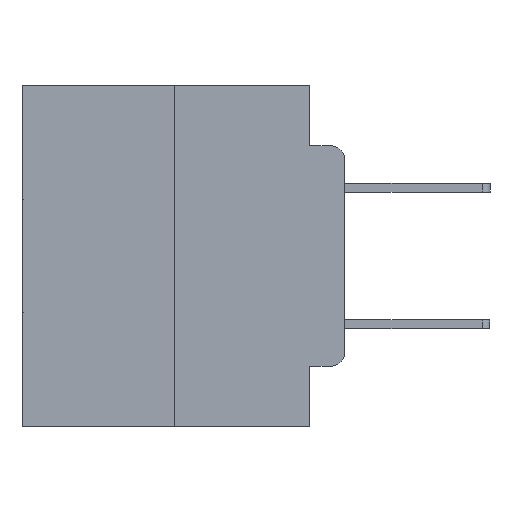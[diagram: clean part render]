
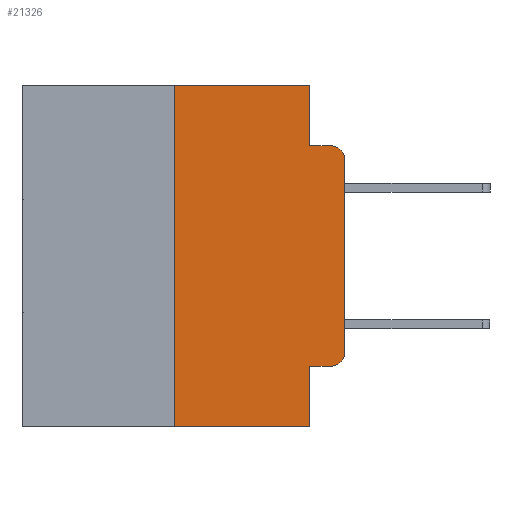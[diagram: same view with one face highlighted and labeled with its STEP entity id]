
A CAD part, left-side view. The second image highlights one B-rep face of the part: STEP entity #21326.
In plain terms, the highlighted planar face has unit normal (-1, 0, 0).
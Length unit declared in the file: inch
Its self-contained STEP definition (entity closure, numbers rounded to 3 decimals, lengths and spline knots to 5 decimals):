
#65 = VECTOR ( 'NONE', #10682, 39.37008 ) ;
#581 = AXIS2_PLACEMENT_3D ( 'NONE', #2863, #18150, #5089 ) ;
#808 = CARTESIAN_POINT ( 'NONE',  ( 0., 0.02, -0.0885 ) ) ;
#842 = CARTESIAN_POINT ( 'NONE',  ( 0., 0.473, 0. ) ) ;
#845 = CARTESIAN_POINT ( 'NONE',  ( 0., 0.051, -0.0885 ) ) ;
#1761 = LINE ( 'NONE', #6382, #12004 ) ;
#1938 = ORIENTED_EDGE ( 'NONE', *, *, #10150, .F. ) ;
#2787 = DIRECTION ( 'NONE',  ( 0., -1., 0. ) ) ;
#2863 = CARTESIAN_POINT ( 'NONE',  ( 0., 0.02, -0.1085 ) ) ;
#3636 = VECTOR ( 'NONE', #24795, 39.37008 ) ;
#4449 = AXIS2_PLACEMENT_3D ( 'NONE', #5507, #20698, #7735 ) ;
#4589 = CARTESIAN_POINT ( 'NONE',  ( 0., 0., -0.3915 ) ) ;
#4652 = VECTOR ( 'NONE', #23548, 39.37008 ) ;
#4990 = EDGE_LOOP ( 'NONE', ( #17980, #5384, #1938, #7462, #9642, #26324, #7247, #12458, #26507, #12456 ) ) ;
#5089 = DIRECTION ( 'NONE',  ( 0., 0., -1. ) ) ;
#5300 = DIRECTION ( 'NONE',  ( 1., 0., 0. ) ) ;
#5384 = ORIENTED_EDGE ( 'NONE', *, *, #11597, .T. ) ;
#5507 = CARTESIAN_POINT ( 'NONE',  ( 0., 0.02, -0.3915 ) ) ;
#5779 = EDGE_CURVE ( 'NONE', #7397, #6292, #14840, .T. ) ;
#6292 = VERTEX_POINT ( 'NONE', #16564 ) ;
#6382 = CARTESIAN_POINT ( 'NONE',  ( 0., 0.473, -0.5 ) ) ;
#6900 = FACE_OUTER_BOUND ( 'NONE', #4990, .T. ) ;
#7247 = ORIENTED_EDGE ( 'NONE', *, *, #27016, .T. ) ;
#7397 = VERTEX_POINT ( 'NONE', #4589 ) ;
#7462 = ORIENTED_EDGE ( 'NONE', *, *, #11059, .F. ) ;
#7468 = DIRECTION ( 'NONE',  ( 0., 0., -1. ) ) ;
#7735 = DIRECTION ( 'NONE',  ( 0., 0., -1. ) ) ;
#8162 = VERTEX_POINT ( 'NONE', #11387 ) ;
#8421 = CARTESIAN_POINT ( 'NONE',  ( 0., 0., 0. ) ) ;
#9582 = PLANE ( 'NONE',  #23136 ) ;
#9642 = ORIENTED_EDGE ( 'NONE', *, *, #26038, .F. ) ;
#9978 = VECTOR ( 'NONE', #7468, 39.37008 ) ;
#10150 = EDGE_CURVE ( 'NONE', #20978, #27968, #14664, .T. ) ;
#10536 = CIRCLE ( 'NONE', #4449, 0.02 ) ;
#10682 = DIRECTION ( 'NONE',  ( 0., -1., 0. ) ) ;
#10781 = VERTEX_POINT ( 'NONE', #15310 ) ;
#11052 = LINE ( 'NONE', #25806, #65 ) ;
#11059 = EDGE_CURVE ( 'NONE', #8162, #20978, #19722, .T. ) ;
#11387 = CARTESIAN_POINT ( 'NONE',  ( 0., 0.051, 0. ) ) ;
#11597 = EDGE_CURVE ( 'NONE', #6292, #27968, #12543, .T. ) ;
#11828 = CARTESIAN_POINT ( 'NONE',  ( 0., 0.25, 0. ) ) ;
#12004 = VECTOR ( 'NONE', #25868, 39.37008 ) ;
#12456 = ORIENTED_EDGE ( 'NONE', *, *, #22674, .T. ) ;
#12458 = ORIENTED_EDGE ( 'NONE', *, *, #19800, .F. ) ;
#12543 = CIRCLE ( 'NONE', #581, 0.02 ) ;
#13041 = EDGE_CURVE ( 'NONE', #10781, #26845, #20321, .T. ) ;
#13046 = DIRECTION ( 'NONE',  ( 0., -1., 0. ) ) ;
#13272 = VERTEX_POINT ( 'NONE', #19242 ) ;
#14606 = VECTOR ( 'NONE', #26967, 39.37008 ) ;
#14664 = LINE ( 'NONE', #15153, #25472 ) ;
#14840 = LINE ( 'NONE', #8421, #4652 ) ;
#15153 = CARTESIAN_POINT ( 'NONE',  ( 0., 0.051, -0.0885 ) ) ;
#15310 = CARTESIAN_POINT ( 'NONE',  ( 0., 0.25, -0.5 ) ) ;
#15766 = LINE ( 'NONE', #20454, #9978 ) ;
#16564 = CARTESIAN_POINT ( 'NONE',  ( 0., 0., -0.1085 ) ) ;
#17858 = CARTESIAN_POINT ( 'NONE',  ( 0., 0.051, -0.4115 ) ) ;
#17980 = ORIENTED_EDGE ( 'NONE', *, *, #5779, .T. ) ;
#18150 = DIRECTION ( 'NONE',  ( -1., 0., 0. ) ) ;
#19242 = CARTESIAN_POINT ( 'NONE',  ( 0., 0.02, -0.4115 ) ) ;
#19722 = LINE ( 'NONE', #24822, #14606 ) ;
#19795 = VECTOR ( 'NONE', #2787, 39.37008 ) ;
#19800 = EDGE_CURVE ( 'NONE', #27847, #20444, #15766, .T. ) ;
#20118 = CARTESIAN_POINT ( 'NONE',  ( 0., 0.051, -0.4115 ) ) ;
#20321 = LINE ( 'NONE', #11828, #3636 ) ;
#20444 = VERTEX_POINT ( 'NONE', #22871 ) ;
#20454 = CARTESIAN_POINT ( 'NONE',  ( 0., 0.051, 0. ) ) ;
#20491 = DIRECTION ( 'NONE',  ( 0., 0., -1. ) ) ;
#20698 = DIRECTION ( 'NONE',  ( -1., 0., 0. ) ) ;
#20978 = VERTEX_POINT ( 'NONE', #845 ) ;
#21247 = EDGE_CURVE ( 'NONE', #27847, #13272, #25498, .T. ) ;
#21326 = ADVANCED_FACE ( 'NONE', ( #6900 ), #9582, .F. ) ;
#22472 = CARTESIAN_POINT ( 'NONE',  ( 0., 0.25, 0. ) ) ;
#22674 = EDGE_CURVE ( 'NONE', #13272, #7397, #10536, .T. ) ;
#22871 = CARTESIAN_POINT ( 'NONE',  ( 0., 0.051, -0.5 ) ) ;
#23136 = AXIS2_PLACEMENT_3D ( 'NONE', #842, #5300, #20491 ) ;
#23548 = DIRECTION ( 'NONE',  ( 0., 0., 1. ) ) ;
#24795 = DIRECTION ( 'NONE',  ( 0., 0., 1. ) ) ;
#24822 = CARTESIAN_POINT ( 'NONE',  ( 0., 0.051, 0. ) ) ;
#25472 = VECTOR ( 'NONE', #13046, 39.37008 ) ;
#25498 = LINE ( 'NONE', #20118, #19795 ) ;
#25806 = CARTESIAN_POINT ( 'NONE',  ( 0., 0.473, 0. ) ) ;
#25868 = DIRECTION ( 'NONE',  ( 0., -1., 0. ) ) ;
#26038 = EDGE_CURVE ( 'NONE', #26845, #8162, #11052, .T. ) ;
#26324 = ORIENTED_EDGE ( 'NONE', *, *, #13041, .F. ) ;
#26507 = ORIENTED_EDGE ( 'NONE', *, *, #21247, .T. ) ;
#26845 = VERTEX_POINT ( 'NONE', #22472 ) ;
#26967 = DIRECTION ( 'NONE',  ( 0., 0., -1. ) ) ;
#27016 = EDGE_CURVE ( 'NONE', #10781, #20444, #1761, .T. ) ;
#27847 = VERTEX_POINT ( 'NONE', #17858 ) ;
#27968 = VERTEX_POINT ( 'NONE', #808 ) ;
